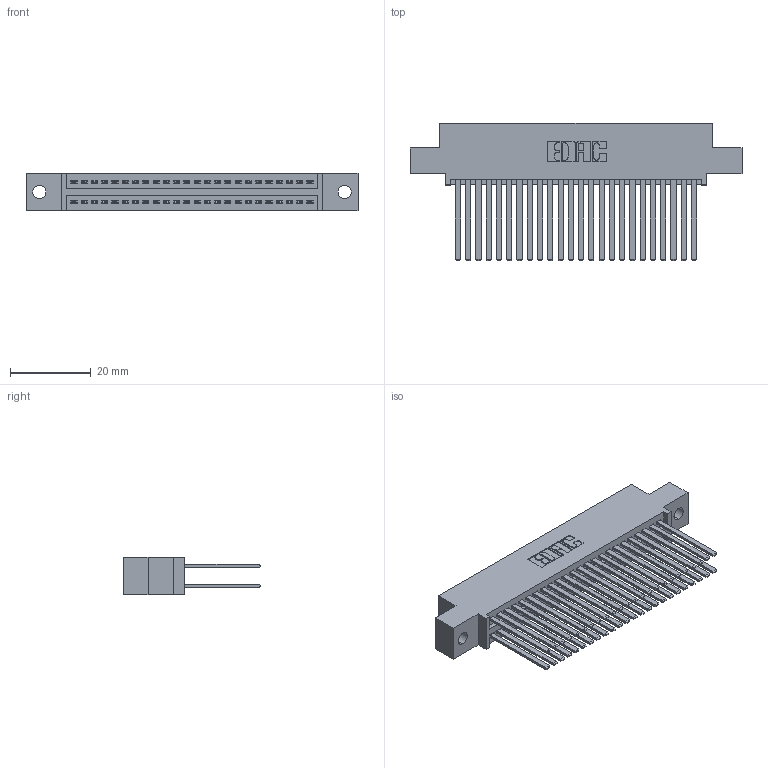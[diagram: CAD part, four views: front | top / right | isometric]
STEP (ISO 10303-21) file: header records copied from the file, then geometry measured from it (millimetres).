
FILE_DESCRIPTION (( 'STEP AP203' ), '1' );
FILE_NAME ('345-048-544-502.STEP', '2019-10-29T05:12:48', ( '' ), ( '' ), 'SwSTEP 2.0', 'SolidWorks 2016', '' );
FILE_SCHEMA (( 'CONFIG_CONTROL_DESIGN' ));
Length unit declared in the file: inch
Products named in the file (3): 345-048-544-502; 345 Part_0.110 Offset - 0.128 Dia; 345-292-001_345-293-144
Assembly tree (49 placements, depth 2):
  345-048-544-502
    345 Part_0.110 Offset - 0.128 Dia
    345-292-001_345-293-144  x48
Bounding box: 82.17 x 33.96 x 9.4 mm (x, y, z)
Volume: 8377.7 mm3; surface area: 13827.3 mm2
Topology: 49 solids, 49 shells, 2242 faces, 6641 edges, 4362 vertices
Faces by surface type: plane 1476, cylinder 766
Entity records: 21205 total; most frequent: CARTESIAN_POINT 3572, ORIENTED_EDGE 3506, DIRECTION 3169, EDGE_CURVE 1753, VECTOR 1529, LINE 1529, VERTEX_POINT 1166, AXIS2_PLACEMENT_3D 820
